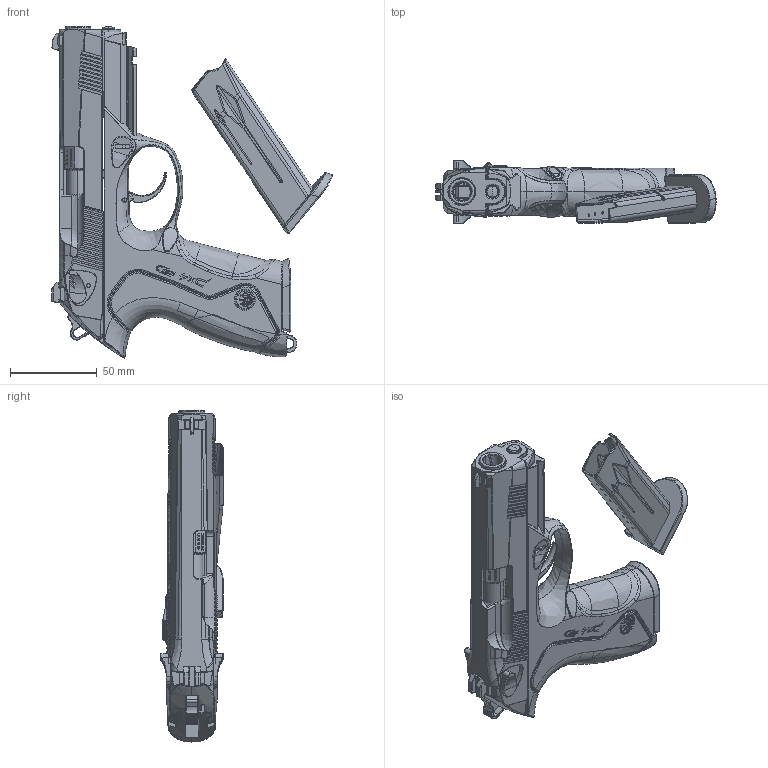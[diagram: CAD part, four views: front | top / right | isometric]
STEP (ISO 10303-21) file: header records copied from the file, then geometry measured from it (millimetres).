
FILE_DESCRIPTION (( 'STEP AP214' ), '1' );
FILE_NAME ('beretta PX4 Storm.STEP', '2019-02-01T15:54:34', ( '' ), ( '' ), 'SwSTEP 2.0', 'SolidWorks 2018', '' );
FILE_SCHEMA (( 'AUTOMOTIVE_DESIGN' ));
Length unit declared in the file: millimetre
Products named in the file (1): beretta PX4 Storm
Bounding box: 161.84 x 36.12 x 191.65 mm (x, y, z)
Volume: 215332.5 mm3; surface area: 116112.4 mm2
Topology: 19 solids, 19 shells, 4887 faces, 12454 edges, 7694 vertices
Faces by surface type: bspline 1870, plane 1624, cylinder 1006, torus 256, sphere 112, cone 19
Entity records: 288470 total; most frequent: CARTESIAN_POINT 187359, ORIENTED_EDGE 24696, DIRECTION 15628, EDGE_CURVE 12348, VERTEX_POINT 7662, AXIS2_PLACEMENT_3D 5608, EDGE_LOOP 5110, ADVANCED_FACE 4885
